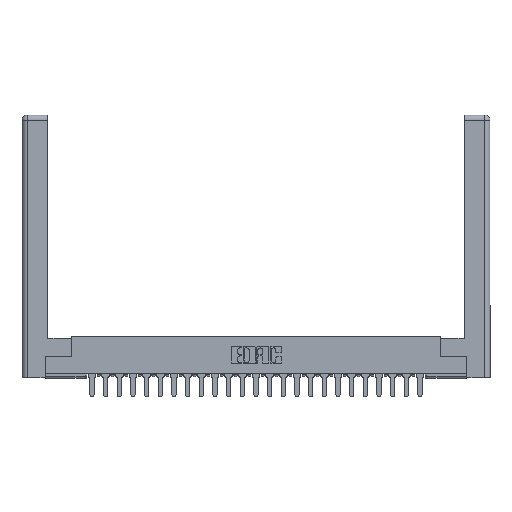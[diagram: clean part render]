
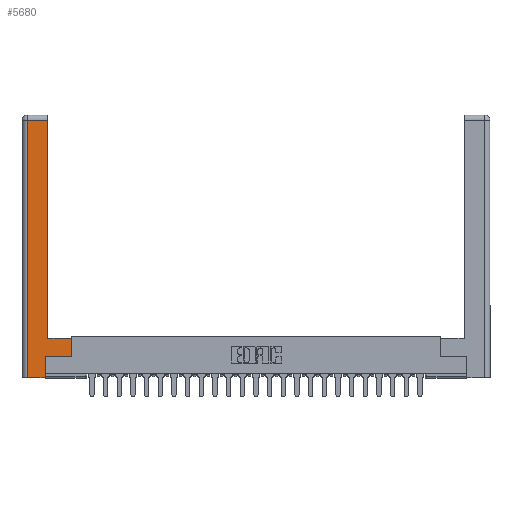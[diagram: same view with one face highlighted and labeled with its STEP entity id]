
A CAD part, top view. The second image highlights one B-rep face of the part: STEP entity #5680.
In plain terms, the highlighted planar face has unit normal (0, 0, 1).
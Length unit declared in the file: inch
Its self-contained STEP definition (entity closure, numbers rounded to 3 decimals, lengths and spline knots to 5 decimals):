
#351 = EDGE_CURVE ( 'NONE', #24953, #8540, #7096, .T. ) ;
#793 = EDGE_CURVE ( 'NONE', #26089, #9805, #2085, .T. ) ;
#2085 = LINE ( 'NONE', #22948, #22529 ) ;
#2159 = VECTOR ( 'NONE', #18546, 39.37008 ) ;
#2991 = PLANE ( 'NONE',  #3186 ) ;
#3128 = DIRECTION ( 'NONE',  ( -1., 0., 0. ) ) ;
#3186 = AXIS2_PLACEMENT_3D ( 'NONE', #5045, #25904, #3128 ) ;
#4229 = LINE ( 'NONE', #24687, #2159 ) ;
#4320 = CARTESIAN_POINT ( 'NONE',  ( 0.265, 0., 0. ) ) ;
#4331 = CARTESIAN_POINT ( 'NONE',  ( 0.295, 0.45, 0. ) ) ;
#5045 = CARTESIAN_POINT ( 'NONE',  ( 0., 0., 0. ) ) ;
#5680 = ADVANCED_FACE ( 'NONE', ( #21813 ), #2991, .F. ) ;
#7096 = LINE ( 'NONE', #23715, #26764 ) ;
#7176 = CARTESIAN_POINT ( 'NONE',  ( 0.0615, 0., 0. ) ) ;
#7585 = ORIENTED_EDGE ( 'NONE', *, *, #12397, .T. ) ;
#7938 = CARTESIAN_POINT ( 'NONE',  ( 0.0615, 0., 0. ) ) ;
#8133 = CARTESIAN_POINT ( 'NONE',  ( 0.295, 0.45, 0. ) ) ;
#8540 = VERTEX_POINT ( 'NONE', #16366 ) ;
#8567 = DIRECTION ( 'NONE',  ( 1., 0., 0. ) ) ;
#8694 = DIRECTION ( 'NONE',  ( 0., -1., 0. ) ) ;
#8845 = LINE ( 'NONE', #4331, #19907 ) ;
#9805 = VERTEX_POINT ( 'NONE', #12887 ) ;
#9910 = ORIENTED_EDGE ( 'NONE', *, *, #10597, .T. ) ;
#10527 = EDGE_CURVE ( 'NONE', #11847, #16805, #12019, .T. ) ;
#10597 = EDGE_CURVE ( 'NONE', #9805, #11847, #15365, .T. ) ;
#11847 = VERTEX_POINT ( 'NONE', #7938 ) ;
#11882 = CARTESIAN_POINT ( 'NONE',  ( 0.265, 0., 0. ) ) ;
#12019 = LINE ( 'NONE', #4320, #22699 ) ;
#12363 = ORIENTED_EDGE ( 'NONE', *, *, #793, .T. ) ;
#12397 = EDGE_CURVE ( 'NONE', #8540, #24782, #8845, .T. ) ;
#12814 = CARTESIAN_POINT ( 'NONE',  ( 0.265, 0.245, 0. ) ) ;
#12887 = CARTESIAN_POINT ( 'NONE',  ( 0.0615, 2.94, 0. ) ) ;
#12944 = CARTESIAN_POINT ( 'NONE',  ( 0.295, 2.94, 0. ) ) ;
#13367 = DIRECTION ( 'NONE',  ( 0., 1., 0. ) ) ;
#13774 = EDGE_LOOP ( 'NONE', ( #25789, #12363, #9910, #18612, #25995, #20768, #24612, #7585 ) ) ;
#14398 = VECTOR ( 'NONE', #21613, 39.37008 ) ;
#15365 = LINE ( 'NONE', #7176, #23545 ) ;
#16366 = CARTESIAN_POINT ( 'NONE',  ( 0.565, 0.45, 0. ) ) ;
#16805 = VERTEX_POINT ( 'NONE', #11882 ) ;
#16852 = CARTESIAN_POINT ( 'NONE',  ( 0.565, 0.245, 0. ) ) ;
#17157 = DIRECTION ( 'NONE',  ( -1., 0., 0. ) ) ;
#18546 = DIRECTION ( 'NONE',  ( 0., 1., 0. ) ) ;
#18612 = ORIENTED_EDGE ( 'NONE', *, *, #10527, .T. ) ;
#18717 = DIRECTION ( 'NONE',  ( -1., 0., 0. ) ) ;
#19470 = LINE ( 'NONE', #12814, #25230 ) ;
#19881 = CARTESIAN_POINT ( 'NONE',  ( 0.265, 0.245, 0. ) ) ;
#19907 = VECTOR ( 'NONE', #17157, 39.37008 ) ;
#20768 = ORIENTED_EDGE ( 'NONE', *, *, #24962, .T. ) ;
#21053 = EDGE_CURVE ( 'NONE', #16805, #26299, #19470, .T. ) ;
#21392 = DIRECTION ( 'NONE',  ( 0., 1., 0. ) ) ;
#21613 = DIRECTION ( 'NONE',  ( 1., 0., 0. ) ) ;
#21813 = FACE_OUTER_BOUND ( 'NONE', #13774, .T. ) ;
#22130 = CARTESIAN_POINT ( 'NONE',  ( 0.565, 0.245, 0. ) ) ;
#22529 = VECTOR ( 'NONE', #18717, 39.37008 ) ;
#22699 = VECTOR ( 'NONE', #8567, 39.37008 ) ;
#22948 = CARTESIAN_POINT ( 'NONE',  ( 0.0615, 2.94, 0. ) ) ;
#23545 = VECTOR ( 'NONE', #8694, 39.37008 ) ;
#23715 = CARTESIAN_POINT ( 'NONE',  ( 0.565, 0.45, 0. ) ) ;
#23864 = EDGE_CURVE ( 'NONE', #24782, #26089, #4229, .T. ) ;
#24612 = ORIENTED_EDGE ( 'NONE', *, *, #351, .T. ) ;
#24687 = CARTESIAN_POINT ( 'NONE',  ( 0.295, 3., 0. ) ) ;
#24782 = VERTEX_POINT ( 'NONE', #8133 ) ;
#24953 = VERTEX_POINT ( 'NONE', #16852 ) ;
#24962 = EDGE_CURVE ( 'NONE', #26299, #24953, #25157, .T. ) ;
#25157 = LINE ( 'NONE', #22130, #14398 ) ;
#25230 = VECTOR ( 'NONE', #21392, 39.37008 ) ;
#25789 = ORIENTED_EDGE ( 'NONE', *, *, #23864, .T. ) ;
#25904 = DIRECTION ( 'NONE',  ( 0., 0., -1. ) ) ;
#25995 = ORIENTED_EDGE ( 'NONE', *, *, #21053, .T. ) ;
#26089 = VERTEX_POINT ( 'NONE', #12944 ) ;
#26299 = VERTEX_POINT ( 'NONE', #19881 ) ;
#26764 = VECTOR ( 'NONE', #13367, 39.37008 ) ;
